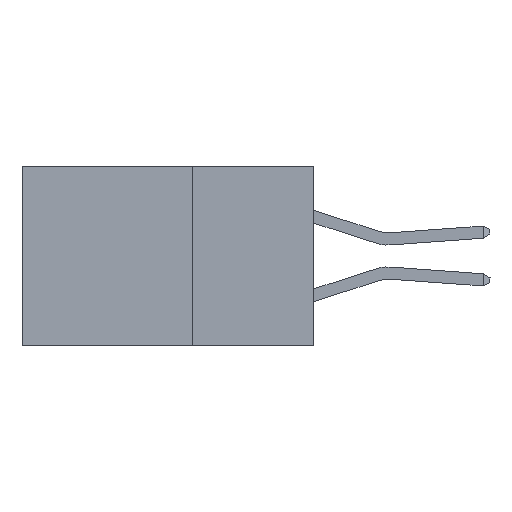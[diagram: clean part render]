
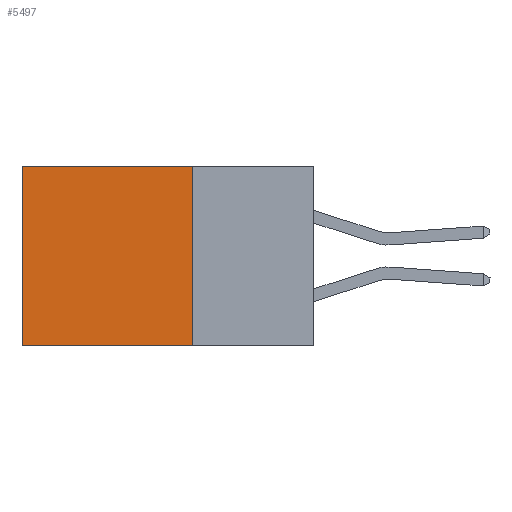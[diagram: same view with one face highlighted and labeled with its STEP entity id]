
A CAD part, left-side view. The second image highlights one B-rep face of the part: STEP entity #5497.
In plain terms, the highlighted planar face has unit normal (-1, 0, 0).
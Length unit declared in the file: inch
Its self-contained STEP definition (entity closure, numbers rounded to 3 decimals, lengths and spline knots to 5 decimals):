
#187 = DIRECTION ( 'NONE',  ( 0., 0., -1. ) ) ;
#1434 = VECTOR ( 'NONE', #5627, 39.37008 ) ;
#1559 = CARTESIAN_POINT ( 'NONE',  ( 0.2875, 0.25, 0. ) ) ;
#1743 = EDGE_CURVE ( 'NONE', #4352, #7102, #3312, .T. ) ;
#1759 = DIRECTION ( 'NONE',  ( 0., 1., 0. ) ) ;
#1769 = PLANE ( 'NONE',  #19027 ) ;
#1893 = ORIENTED_EDGE ( 'NONE', *, *, #3125, .T. ) ;
#3125 = EDGE_CURVE ( 'NONE', #4352, #14307, #5247, .T. ) ;
#3312 = LINE ( 'NONE', #19555, #20284 ) ;
#4208 = CARTESIAN_POINT ( 'NONE',  ( 0.2875, 0.6, -0.37 ) ) ;
#4352 = VERTEX_POINT ( 'NONE', #1559 ) ;
#4522 = CARTESIAN_POINT ( 'NONE',  ( 0.2875, 0.25, -0.37 ) ) ;
#5168 = FACE_OUTER_BOUND ( 'NONE', #9630, .T. ) ;
#5247 = LINE ( 'NONE', #11585, #18409 ) ;
#5497 = ADVANCED_FACE ( 'NONE', ( #5168 ), #1769, .F. ) ;
#5627 = DIRECTION ( 'NONE',  ( 0., 1., 0. ) ) ;
#5801 = LINE ( 'NONE', #8874, #1434 ) ;
#6041 = ORIENTED_EDGE ( 'NONE', *, *, #19928, .F. ) ;
#7102 = VERTEX_POINT ( 'NONE', #4522 ) ;
#8726 = EDGE_CURVE ( 'NONE', #14307, #11843, #15041, .T. ) ;
#8779 = CARTESIAN_POINT ( 'NONE',  ( 0.2875, 0.6, 0. ) ) ;
#8874 = CARTESIAN_POINT ( 'NONE',  ( 0.2875, 0.25, -0.37 ) ) ;
#9630 = EDGE_LOOP ( 'NONE', ( #13135, #6041, #18003, #1893 ) ) ;
#9924 = DIRECTION ( 'NONE',  ( 0., 0., -1. ) ) ;
#10009 = DIRECTION ( 'NONE',  ( 1., 0., 0. ) ) ;
#11585 = CARTESIAN_POINT ( 'NONE',  ( 0.2875, 0.25, 0. ) ) ;
#11843 = VERTEX_POINT ( 'NONE', #4208 ) ;
#13135 = ORIENTED_EDGE ( 'NONE', *, *, #8726, .T. ) ;
#13214 = CARTESIAN_POINT ( 'NONE',  ( 0.2875, 0.6, 0. ) ) ;
#14307 = VERTEX_POINT ( 'NONE', #8779 ) ;
#14515 = VECTOR ( 'NONE', #9924, 39.37008 ) ;
#15041 = LINE ( 'NONE', #13214, #14515 ) ;
#18003 = ORIENTED_EDGE ( 'NONE', *, *, #1743, .F. ) ;
#18409 = VECTOR ( 'NONE', #1759, 39.37008 ) ;
#19027 = AXIS2_PLACEMENT_3D ( 'NONE', #19905, #10009, #187 ) ;
#19555 = CARTESIAN_POINT ( 'NONE',  ( 0.2875, 0.25, 0. ) ) ;
#19625 = DIRECTION ( 'NONE',  ( 0., 0., -1. ) ) ;
#19905 = CARTESIAN_POINT ( 'NONE',  ( 0.2875, 0.25, 0. ) ) ;
#19928 = EDGE_CURVE ( 'NONE', #7102, #11843, #5801, .T. ) ;
#20284 = VECTOR ( 'NONE', #19625, 39.37008 ) ;
